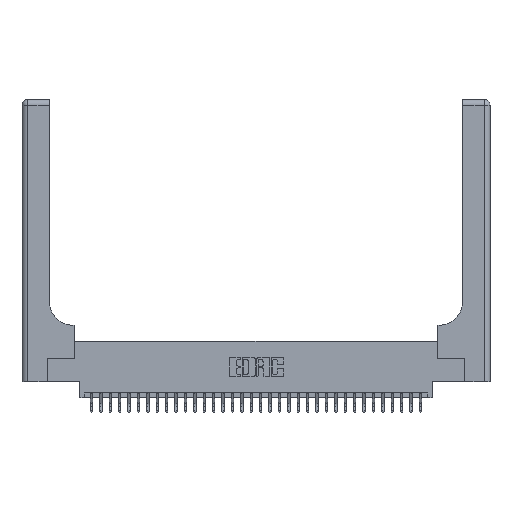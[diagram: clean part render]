
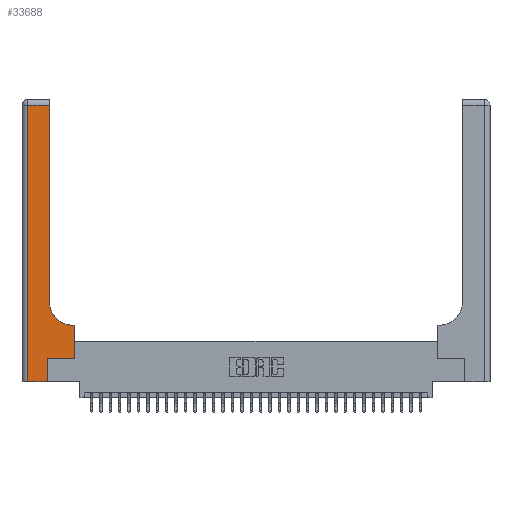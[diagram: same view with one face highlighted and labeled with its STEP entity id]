
A CAD part, top view. The second image highlights one B-rep face of the part: STEP entity #33688.
In plain terms, the highlighted planar face has unit normal (0, 0, 1).
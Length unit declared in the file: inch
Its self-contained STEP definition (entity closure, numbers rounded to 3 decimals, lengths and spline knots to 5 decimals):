
#33 = CARTESIAN_POINT ( 'NONE',  ( 0.269, 0., 0.37 ) ) ;
#581 = EDGE_CURVE ( 'NONE', #7773, #33536, #10225, .T. ) ;
#618 = CARTESIAN_POINT ( 'NONE',  ( 0.2915, 3., 0.37 ) ) ;
#941 = DIRECTION ( 'NONE',  ( 1., 0., 0. ) ) ;
#1062 = CARTESIAN_POINT ( 'NONE',  ( 0.2915, 0.85, 0.37 ) ) ;
#1358 = VECTOR ( 'NONE', #8753, 39.37008 ) ;
#1462 = VERTEX_POINT ( 'NONE', #24633 ) ;
#2027 = CARTESIAN_POINT ( 'NONE',  ( 0., 3., 0.37 ) ) ;
#2867 = EDGE_CURVE ( 'NONE', #29322, #27211, #19682, .T. ) ;
#3101 = VECTOR ( 'NONE', #23859, 39.37008 ) ;
#3356 = ORIENTED_EDGE ( 'NONE', *, *, #32290, .T. ) ;
#4731 = CARTESIAN_POINT ( 'NONE',  ( 0.06, 2.94, 0.37 ) ) ;
#4758 = DIRECTION ( 'NONE',  ( -1., 0., 0. ) ) ;
#5419 = CARTESIAN_POINT ( 'NONE',  ( 0.5415, 0.85, 0.37 ) ) ;
#6589 = DIRECTION ( 'NONE',  ( -1., 0., 0. ) ) ;
#7159 = AXIS2_PLACEMENT_3D ( 'NONE', #2027, #20691, #4758 ) ;
#7292 = EDGE_CURVE ( 'NONE', #15895, #17711, #27884, .T. ) ;
#7773 = VERTEX_POINT ( 'NONE', #20958 ) ;
#7780 = VECTOR ( 'NONE', #21925, 39.37008 ) ;
#7927 = CARTESIAN_POINT ( 'NONE',  ( 0.5585, 0.25, 0.37 ) ) ;
#8095 = DIRECTION ( 'NONE',  ( 1., 0., 0. ) ) ;
#8428 = ORIENTED_EDGE ( 'NONE', *, *, #2867, .T. ) ;
#8753 = DIRECTION ( 'NONE',  ( 0., 1., 0. ) ) ;
#9432 = CARTESIAN_POINT ( 'NONE',  ( 0.5585, 0.6, 0.37 ) ) ;
#9804 = EDGE_CURVE ( 'NONE', #17711, #1462, #16443, .T. ) ;
#10225 = LINE ( 'NONE', #7927, #3101 ) ;
#10550 = DIRECTION ( 'NONE',  ( 0., -1., 0. ) ) ;
#11003 = CARTESIAN_POINT ( 'NONE',  ( 0.269, 0.25, 0.37 ) ) ;
#12155 = ORIENTED_EDGE ( 'NONE', *, *, #17672, .T. ) ;
#13346 = CARTESIAN_POINT ( 'NONE',  ( 0.269, 0., 0.37 ) ) ;
#14817 = EDGE_CURVE ( 'NONE', #33536, #15895, #27495, .T. ) ;
#15684 = LINE ( 'NONE', #24776, #29004 ) ;
#15895 = VERTEX_POINT ( 'NONE', #18801 ) ;
#16443 = LINE ( 'NONE', #618, #1358 ) ;
#16622 = CARTESIAN_POINT ( 'NONE',  ( 0.269, 0.25, 0.37 ) ) ;
#16735 = ORIENTED_EDGE ( 'NONE', *, *, #9804, .T. ) ;
#17199 = ORIENTED_EDGE ( 'NONE', *, *, #581, .T. ) ;
#17383 = FACE_OUTER_BOUND ( 'NONE', #34367, .T. ) ;
#17672 = EDGE_CURVE ( 'NONE', #27213, #29322, #15684, .T. ) ;
#17711 = VERTEX_POINT ( 'NONE', #1062 ) ;
#18017 = EDGE_CURVE ( 'NONE', #26980, #27213, #26882, .T. ) ;
#18801 = CARTESIAN_POINT ( 'NONE',  ( 0.5415, 0.6, 0.37 ) ) ;
#19682 = LINE ( 'NONE', #13346, #26780 ) ;
#19785 = VECTOR ( 'NONE', #10550, 39.37008 ) ;
#20025 = VECTOR ( 'NONE', #6589, 39.37008 ) ;
#20130 = CARTESIAN_POINT ( 'NONE',  ( 0.2915, 0.6, 0.37 ) ) ;
#20379 = VECTOR ( 'NONE', #22789, 39.37008 ) ;
#20691 = DIRECTION ( 'NONE',  ( 0., 0., -1. ) ) ;
#20958 = CARTESIAN_POINT ( 'NONE',  ( 0.5585, 0.25, 0.37 ) ) ;
#21925 = DIRECTION ( 'NONE',  ( 1., 0., 0. ) ) ;
#22570 = ORIENTED_EDGE ( 'NONE', *, *, #23308, .T. ) ;
#22789 = DIRECTION ( 'NONE',  ( -1., 0., 0. ) ) ;
#23308 = EDGE_CURVE ( 'NONE', #27211, #7773, #29873, .T. ) ;
#23859 = DIRECTION ( 'NONE',  ( 0., 1., 0. ) ) ;
#23907 = DIRECTION ( 'NONE',  ( 0., 1., 0. ) ) ;
#24017 = DIRECTION ( 'NONE',  ( 0., 0., -1. ) ) ;
#24633 = CARTESIAN_POINT ( 'NONE',  ( 0.2915, 2.94, 0.37 ) ) ;
#24776 = CARTESIAN_POINT ( 'NONE',  ( 0., 0., 0.37 ) ) ;
#25044 = AXIS2_PLACEMENT_3D ( 'NONE', #5419, #24017, #8095 ) ;
#25221 = CARTESIAN_POINT ( 'NONE',  ( 0., 2.94, 0.37 ) ) ;
#26780 = VECTOR ( 'NONE', #23907, 39.37008 ) ;
#26882 = LINE ( 'NONE', #29194, #19785 ) ;
#26980 = VERTEX_POINT ( 'NONE', #4731 ) ;
#27211 = VERTEX_POINT ( 'NONE', #11003 ) ;
#27213 = VERTEX_POINT ( 'NONE', #29655 ) ;
#27495 = LINE ( 'NONE', #20130, #20379 ) ;
#27884 = CIRCLE ( 'NONE', #25044, 0.25 ) ;
#29004 = VECTOR ( 'NONE', #941, 39.37008 ) ;
#29194 = CARTESIAN_POINT ( 'NONE',  ( 0.06, 3., 0.37 ) ) ;
#29322 = VERTEX_POINT ( 'NONE', #33 ) ;
#29655 = CARTESIAN_POINT ( 'NONE',  ( 0.06, 0., 0.37 ) ) ;
#29873 = LINE ( 'NONE', #16622, #7780 ) ;
#31225 = PLANE ( 'NONE',  #7159 ) ;
#31380 = ORIENTED_EDGE ( 'NONE', *, *, #14817, .T. ) ;
#32290 = EDGE_CURVE ( 'NONE', #1462, #26980, #34230, .T. ) ;
#32564 = ORIENTED_EDGE ( 'NONE', *, *, #18017, .T. ) ;
#33044 = ORIENTED_EDGE ( 'NONE', *, *, #7292, .T. ) ;
#33536 = VERTEX_POINT ( 'NONE', #9432 ) ;
#33688 = ADVANCED_FACE ( 'NONE', ( #17383 ), #31225, .F. ) ;
#34230 = LINE ( 'NONE', #25221, #20025 ) ;
#34367 = EDGE_LOOP ( 'NONE', ( #16735, #3356, #32564, #12155, #8428, #22570, #17199, #31380, #33044 ) ) ;
